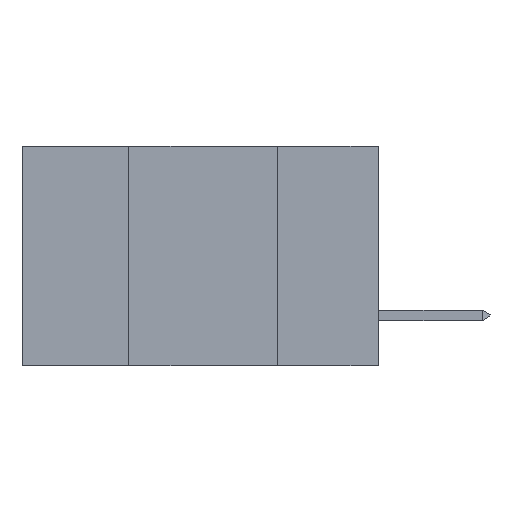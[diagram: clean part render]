
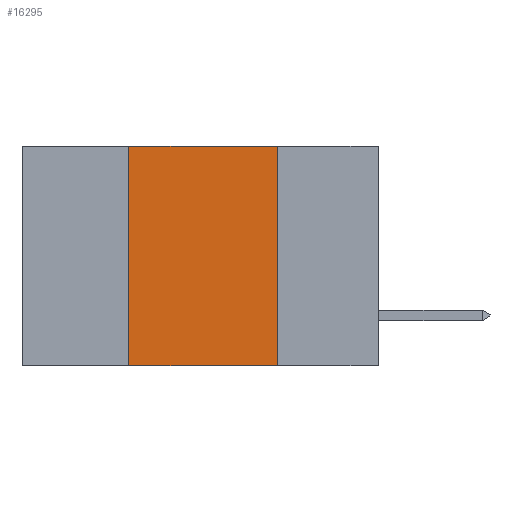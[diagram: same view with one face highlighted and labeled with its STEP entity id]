
A CAD part, left-side view. The second image highlights one B-rep face of the part: STEP entity #16295.
In plain terms, the highlighted planar face has unit normal (-1, 0, 0).
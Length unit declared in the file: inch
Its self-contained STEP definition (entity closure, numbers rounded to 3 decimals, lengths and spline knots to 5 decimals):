
#1602 = VECTOR ( 'NONE', #14210, 39.37008 ) ;
#1825 = EDGE_CURVE ( 'NONE', #5655, #10542, #3975, .T. ) ;
#2505 = EDGE_CURVE ( 'NONE', #11258, #5655, #5694, .T. ) ;
#2876 = CARTESIAN_POINT ( 'NONE',  ( 0., 0.6, -0.37 ) ) ;
#3086 = ORIENTED_EDGE ( 'NONE', *, *, #2505, .F. ) ;
#3191 = EDGE_LOOP ( 'NONE', ( #3444, #9706, #3086, #16608 ) ) ;
#3327 = VERTEX_POINT ( 'NONE', #13438 ) ;
#3444 = ORIENTED_EDGE ( 'NONE', *, *, #6798, .F. ) ;
#3503 = LINE ( 'NONE', #2876, #13487 ) ;
#3819 = DIRECTION ( 'NONE',  ( 0., 0., -1. ) ) ;
#3975 = LINE ( 'NONE', #12707, #1602 ) ;
#4128 = EDGE_CURVE ( 'NONE', #11258, #3327, #3503, .T. ) ;
#5245 = CARTESIAN_POINT ( 'NONE',  ( 0., 0.42, 0. ) ) ;
#5655 = VERTEX_POINT ( 'NONE', #5245 ) ;
#5694 = LINE ( 'NONE', #8885, #7467 ) ;
#6798 = EDGE_CURVE ( 'NONE', #10542, #3327, #10573, .T. ) ;
#6817 = CARTESIAN_POINT ( 'NONE',  ( 0., 0.17, 0. ) ) ;
#6820 = PLANE ( 'NONE',  #10585 ) ;
#6860 = CARTESIAN_POINT ( 'NONE',  ( 0., 0.42, -0.37 ) ) ;
#7467 = VECTOR ( 'NONE', #10282, 39.37008 ) ;
#8167 = CARTESIAN_POINT ( 'NONE',  ( 0., 0.6, 0. ) ) ;
#8630 = VECTOR ( 'NONE', #3819, 39.37008 ) ;
#8885 = CARTESIAN_POINT ( 'NONE',  ( 0., 0.42, 0. ) ) ;
#9538 = DIRECTION ( 'NONE',  ( 0., 0., -1. ) ) ;
#9706 = ORIENTED_EDGE ( 'NONE', *, *, #1825, .F. ) ;
#9727 = FACE_OUTER_BOUND ( 'NONE', #3191, .T. ) ;
#10282 = DIRECTION ( 'NONE',  ( 0., 0., 1. ) ) ;
#10542 = VERTEX_POINT ( 'NONE', #6817 ) ;
#10573 = LINE ( 'NONE', #13381, #8630 ) ;
#10585 = AXIS2_PLACEMENT_3D ( 'NONE', #8167, #17837, #9538 ) ;
#11258 = VERTEX_POINT ( 'NONE', #6860 ) ;
#12707 = CARTESIAN_POINT ( 'NONE',  ( 0., 0.6, 0. ) ) ;
#13381 = CARTESIAN_POINT ( 'NONE',  ( 0., 0.17, 0. ) ) ;
#13438 = CARTESIAN_POINT ( 'NONE',  ( 0., 0.17, -0.37 ) ) ;
#13487 = VECTOR ( 'NONE', #15002, 39.37008 ) ;
#14210 = DIRECTION ( 'NONE',  ( 0., -1., 0. ) ) ;
#15002 = DIRECTION ( 'NONE',  ( 0., -1., 0. ) ) ;
#16295 = ADVANCED_FACE ( 'NONE', ( #9727 ), #6820, .F. ) ;
#16608 = ORIENTED_EDGE ( 'NONE', *, *, #4128, .T. ) ;
#17837 = DIRECTION ( 'NONE',  ( 1., 0., 0. ) ) ;
